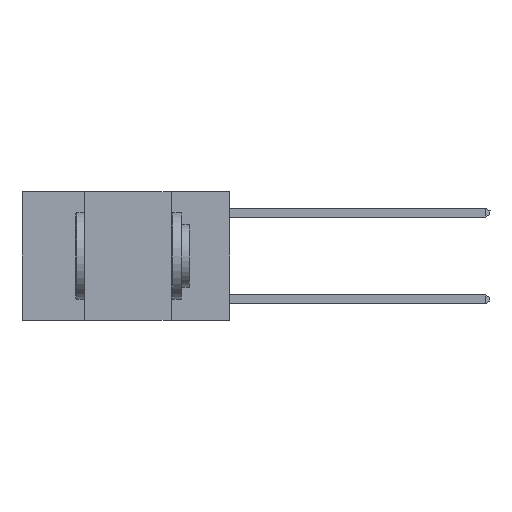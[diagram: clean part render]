
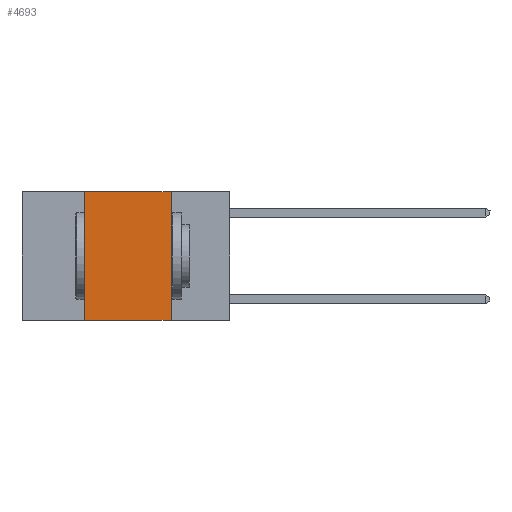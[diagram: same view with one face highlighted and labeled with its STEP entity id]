
A CAD part, left-side view. The second image highlights one B-rep face of the part: STEP entity #4693.
In plain terms, the highlighted planar face has unit normal (-1, 0, 0).
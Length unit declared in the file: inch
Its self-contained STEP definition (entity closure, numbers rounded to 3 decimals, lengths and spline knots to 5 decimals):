
#65 = DIRECTION ( 'NONE',  ( 0., -1., 0. ) ) ;
#950 = LINE ( 'NONE', #15657, #7481 ) ;
#1168 = CARTESIAN_POINT ( 'NONE',  ( 0., 0.42, -0.37 ) ) ;
#1357 = DIRECTION ( 'NONE',  ( 0., 0., -1. ) ) ;
#1378 = LINE ( 'NONE', #9131, #4908 ) ;
#2030 = PLANE ( 'NONE',  #14649 ) ;
#2190 = EDGE_CURVE ( 'NONE', #4651, #14601, #6799, .T. ) ;
#3386 = DIRECTION ( 'NONE',  ( 0., 0., -1. ) ) ;
#4271 = VERTEX_POINT ( 'NONE', #1168 ) ;
#4623 = EDGE_LOOP ( 'NONE', ( #13241, #10432, #16674, #14860 ) ) ;
#4651 = VERTEX_POINT ( 'NONE', #5874 ) ;
#4693 = ADVANCED_FACE ( 'NONE', ( #13178 ), #2030, .F. ) ;
#4908 = VECTOR ( 'NONE', #1357, 39.37008 ) ;
#5673 = VERTEX_POINT ( 'NONE', #15943 ) ;
#5874 = CARTESIAN_POINT ( 'NONE',  ( 0., 0.42, 0. ) ) ;
#5999 = EDGE_CURVE ( 'NONE', #4271, #4651, #10858, .T. ) ;
#6799 = LINE ( 'NONE', #7090, #10615 ) ;
#7090 = CARTESIAN_POINT ( 'NONE',  ( 0., 0.6, 0. ) ) ;
#7481 = VECTOR ( 'NONE', #65, 39.37008 ) ;
#8476 = CARTESIAN_POINT ( 'NONE',  ( 0., 0.6, 0. ) ) ;
#9131 = CARTESIAN_POINT ( 'NONE',  ( 0., 0.17, 0. ) ) ;
#9718 = EDGE_CURVE ( 'NONE', #14601, #5673, #1378, .T. ) ;
#9743 = EDGE_CURVE ( 'NONE', #4271, #5673, #950, .T. ) ;
#10060 = DIRECTION ( 'NONE',  ( 0., 0., 1. ) ) ;
#10432 = ORIENTED_EDGE ( 'NONE', *, *, #2190, .F. ) ;
#10440 = VECTOR ( 'NONE', #10060, 39.37008 ) ;
#10615 = VECTOR ( 'NONE', #16147, 39.37008 ) ;
#10858 = LINE ( 'NONE', #16614, #10440 ) ;
#11093 = DIRECTION ( 'NONE',  ( 1., 0., 0. ) ) ;
#13178 = FACE_OUTER_BOUND ( 'NONE', #4623, .T. ) ;
#13241 = ORIENTED_EDGE ( 'NONE', *, *, #9718, .F. ) ;
#14601 = VERTEX_POINT ( 'NONE', #14652 ) ;
#14649 = AXIS2_PLACEMENT_3D ( 'NONE', #8476, #11093, #3386 ) ;
#14652 = CARTESIAN_POINT ( 'NONE',  ( 0., 0.17, 0. ) ) ;
#14860 = ORIENTED_EDGE ( 'NONE', *, *, #9743, .T. ) ;
#15657 = CARTESIAN_POINT ( 'NONE',  ( 0., 0.6, -0.37 ) ) ;
#15943 = CARTESIAN_POINT ( 'NONE',  ( 0., 0.17, -0.37 ) ) ;
#16147 = DIRECTION ( 'NONE',  ( 0., -1., 0. ) ) ;
#16614 = CARTESIAN_POINT ( 'NONE',  ( 0., 0.42, 0. ) ) ;
#16674 = ORIENTED_EDGE ( 'NONE', *, *, #5999, .F. ) ;
